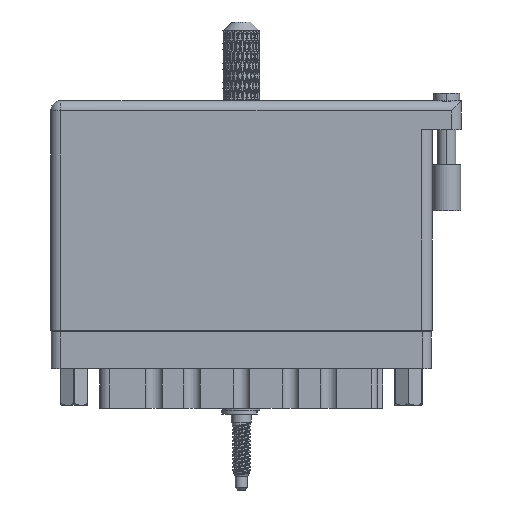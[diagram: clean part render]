
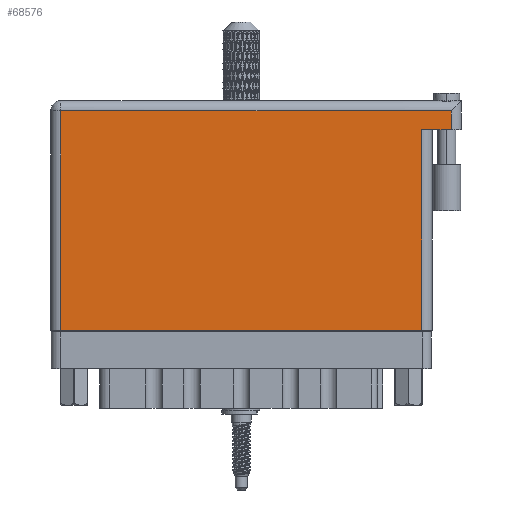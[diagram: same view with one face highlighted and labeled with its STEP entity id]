
A CAD part, front view. The second image highlights one B-rep face of the part: STEP entity #68576.
In plain terms, the highlighted face is planar.
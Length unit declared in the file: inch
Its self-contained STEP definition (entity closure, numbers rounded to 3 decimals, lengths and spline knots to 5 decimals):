
#1143 = CARTESIAN_POINT ( 'NONE',  ( 2.53, 1.369, 0. ) ) ;
#5015 = VECTOR ( 'NONE', #106802, 39.37008 ) ;
#8694 = CARTESIAN_POINT ( 'NONE',  ( 2.73, 1.369, 0. ) ) ;
#10546 = DIRECTION ( 'NONE',  ( -1., 0., 0. ) ) ;
#11189 = ORIENTED_EDGE ( 'NONE', *, *, #20452, .T. ) ;
#11317 = VERTEX_POINT ( 'NONE', #79339 ) ;
#12069 = EDGE_CURVE ( 'NONE', #11317, #81291, #116482, .T. ) ;
#16860 = AXIS2_PLACEMENT_3D ( 'NONE', #69055, #49178, #116796 ) ;
#20452 = EDGE_CURVE ( 'NONE', #35242, #99648, #101781, .T. ) ;
#22013 = DIRECTION ( 'NONE',  ( 0., -1., 0. ) ) ;
#28640 = VECTOR ( 'NONE', #114863, 39.37008 ) ;
#29370 = VECTOR ( 'NONE', #22013, 39.37008 ) ;
#31107 = LINE ( 'NONE', #70063, #41453 ) ;
#35242 = VERTEX_POINT ( 'NONE', #95571 ) ;
#36801 = CARTESIAN_POINT ( 'NONE',  ( 0., 1.496, 0. ) ) ;
#37499 = EDGE_CURVE ( 'NONE', #73272, #11317, #31107, .T. ) ;
#39264 = CARTESIAN_POINT ( 'NONE',  ( 2.8, 1.369, 0. ) ) ;
#41453 = VECTOR ( 'NONE', #52268, 39.37008 ) ;
#49178 = DIRECTION ( 'NONE',  ( 0., 0., -1. ) ) ;
#49375 = LINE ( 'NONE', #120769, #58301 ) ;
#49552 = CARTESIAN_POINT ( 'NONE',  ( 2.53, 1.369, 0. ) ) ;
#50162 = EDGE_CURVE ( 'NONE', #74716, #35242, #49375, .T. ) ;
#50416 = PLANE ( 'NONE',  #16860 ) ;
#52268 = DIRECTION ( 'NONE',  ( 1., 0., 0. ) ) ;
#56117 = LINE ( 'NONE', #76826, #29370 ) ;
#56925 = LINE ( 'NONE', #39264, #28640 ) ;
#58090 = ORIENTED_EDGE ( 'NONE', *, *, #104183, .T. ) ;
#58301 = VECTOR ( 'NONE', #65863, 39.37008 ) ;
#65863 = DIRECTION ( 'NONE',  ( 0., 1., 0. ) ) ;
#68576 = ADVANCED_FACE ( 'NONE', ( #78365 ), #50416, .F. ) ;
#69055 = CARTESIAN_POINT ( 'NONE',  ( 0., 1.566, 0. ) ) ;
#70063 = CARTESIAN_POINT ( 'NONE',  ( 0., 0., 0. ) ) ;
#72549 = CARTESIAN_POINT ( 'NONE',  ( 0.07, 0., 0. ) ) ;
#73272 = VERTEX_POINT ( 'NONE', #72549 ) ;
#74716 = VERTEX_POINT ( 'NONE', #8694 ) ;
#76826 = CARTESIAN_POINT ( 'NONE',  ( 0.07, 0., 0. ) ) ;
#78365 = FACE_OUTER_BOUND ( 'NONE', #88661, .T. ) ;
#79339 = CARTESIAN_POINT ( 'NONE',  ( 2.53, 0., 0. ) ) ;
#81291 = VERTEX_POINT ( 'NONE', #1143 ) ;
#82498 = VECTOR ( 'NONE', #10546, 39.37008 ) ;
#88661 = EDGE_LOOP ( 'NONE', ( #96399, #116661, #93237, #115147, #11189, #58090 ) ) ;
#93237 = ORIENTED_EDGE ( 'NONE', *, *, #98673, .F. ) ;
#95571 = CARTESIAN_POINT ( 'NONE',  ( 2.73, 1.496, 0. ) ) ;
#96399 = ORIENTED_EDGE ( 'NONE', *, *, #37499, .T. ) ;
#98659 = CARTESIAN_POINT ( 'NONE',  ( 0.07, 1.496, 0. ) ) ;
#98673 = EDGE_CURVE ( 'NONE', #74716, #81291, #56925, .T. ) ;
#99648 = VERTEX_POINT ( 'NONE', #98659 ) ;
#101781 = LINE ( 'NONE', #36801, #82498 ) ;
#104183 = EDGE_CURVE ( 'NONE', #99648, #73272, #56117, .T. ) ;
#106802 = DIRECTION ( 'NONE',  ( 0., 1., 0. ) ) ;
#114863 = DIRECTION ( 'NONE',  ( -1., 0., 0. ) ) ;
#115147 = ORIENTED_EDGE ( 'NONE', *, *, #50162, .T. ) ;
#116482 = LINE ( 'NONE', #49552, #5015 ) ;
#116661 = ORIENTED_EDGE ( 'NONE', *, *, #12069, .T. ) ;
#116796 = DIRECTION ( 'NONE',  ( -1., 0., 0. ) ) ;
#120769 = CARTESIAN_POINT ( 'NONE',  ( 2.73, 1.566, 0. ) ) ;
